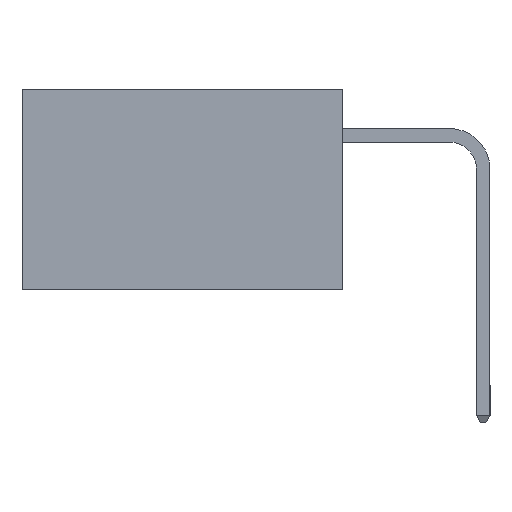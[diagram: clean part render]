
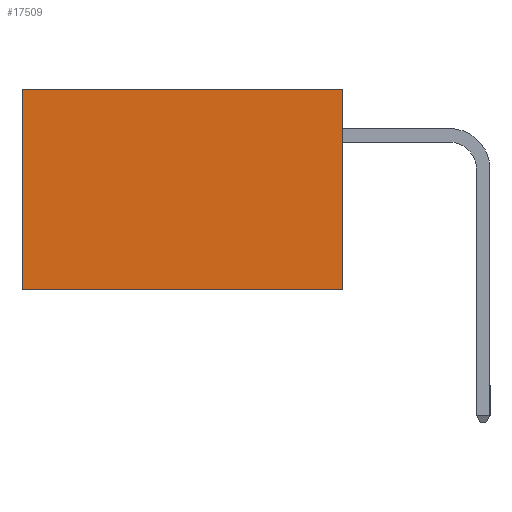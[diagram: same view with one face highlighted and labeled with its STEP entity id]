
A CAD part, left-side view. The second image highlights one B-rep face of the part: STEP entity #17509.
In plain terms, the highlighted planar face has unit normal (-1, 0, 0).
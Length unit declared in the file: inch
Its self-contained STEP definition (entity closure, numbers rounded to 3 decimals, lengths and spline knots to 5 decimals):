
#224 = VECTOR ( 'NONE', #9798, 39.37008 ) ;
#678 = LINE ( 'NONE', #11146, #224 ) ;
#1317 = ORIENTED_EDGE ( 'NONE', *, *, #13159, .T. ) ;
#1375 = VECTOR ( 'NONE', #16448, 39.37008 ) ;
#1396 = ORIENTED_EDGE ( 'NONE', *, *, #8546, .F. ) ;
#2642 = VERTEX_POINT ( 'NONE', #8582 ) ;
#3310 = VERTEX_POINT ( 'NONE', #16957 ) ;
#3902 = EDGE_CURVE ( 'NONE', #2642, #3310, #11672, .T. ) ;
#4911 = DIRECTION ( 'NONE',  ( 0., 0., -1. ) ) ;
#4935 = CARTESIAN_POINT ( 'NONE',  ( 0.277, 0., -0.37 ) ) ;
#5014 = ORIENTED_EDGE ( 'NONE', *, *, #3902, .T. ) ;
#5017 = LINE ( 'NONE', #6844, #1375 ) ;
#6844 = CARTESIAN_POINT ( 'NONE',  ( 0.277, 0., -0.37 ) ) ;
#7252 = CARTESIAN_POINT ( 'NONE',  ( 0.277, 0., -0.37 ) ) ;
#8546 = EDGE_CURVE ( 'NONE', #2642, #15248, #10447, .T. ) ;
#8582 = CARTESIAN_POINT ( 'NONE',  ( 0.277, 0., 0. ) ) ;
#8614 = DIRECTION ( 'NONE',  ( 0., 0., -1. ) ) ;
#8894 = DIRECTION ( 'NONE',  ( 0., 1., 0. ) ) ;
#9236 = FACE_OUTER_BOUND ( 'NONE', #15952, .T. ) ;
#9724 = CARTESIAN_POINT ( 'NONE',  ( 0.277, 0.59, -0.37 ) ) ;
#9798 = DIRECTION ( 'NONE',  ( 0., 0., -1. ) ) ;
#10447 = LINE ( 'NONE', #4935, #13234 ) ;
#11146 = CARTESIAN_POINT ( 'NONE',  ( 0.277, 0.59, -0.37 ) ) ;
#11212 = CARTESIAN_POINT ( 'NONE',  ( 0.277, 0., -0.37 ) ) ;
#11272 = PLANE ( 'NONE',  #17472 ) ;
#11672 = LINE ( 'NONE', #16838, #14856 ) ;
#12166 = ORIENTED_EDGE ( 'NONE', *, *, #17369, .F. ) ;
#13159 = EDGE_CURVE ( 'NONE', #3310, #14199, #678, .T. ) ;
#13234 = VECTOR ( 'NONE', #4911, 39.37008 ) ;
#14199 = VERTEX_POINT ( 'NONE', #9724 ) ;
#14856 = VECTOR ( 'NONE', #8894, 39.37008 ) ;
#15248 = VERTEX_POINT ( 'NONE', #11212 ) ;
#15952 = EDGE_LOOP ( 'NONE', ( #1317, #12166, #1396, #5014 ) ) ;
#16448 = DIRECTION ( 'NONE',  ( 0., 1., 0. ) ) ;
#16728 = DIRECTION ( 'NONE',  ( 1., 0., 0. ) ) ;
#16838 = CARTESIAN_POINT ( 'NONE',  ( 0.277, 0., 0. ) ) ;
#16957 = CARTESIAN_POINT ( 'NONE',  ( 0.277, 0.59, 0. ) ) ;
#17369 = EDGE_CURVE ( 'NONE', #15248, #14199, #5017, .T. ) ;
#17472 = AXIS2_PLACEMENT_3D ( 'NONE', #7252, #16728, #8614 ) ;
#17509 = ADVANCED_FACE ( 'NONE', ( #9236 ), #11272, .F. ) ;
